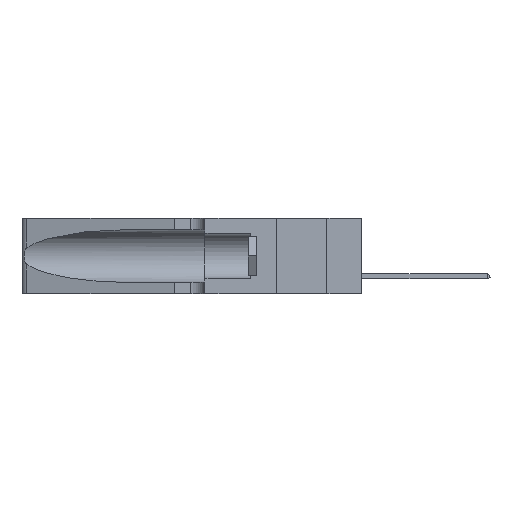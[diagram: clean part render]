
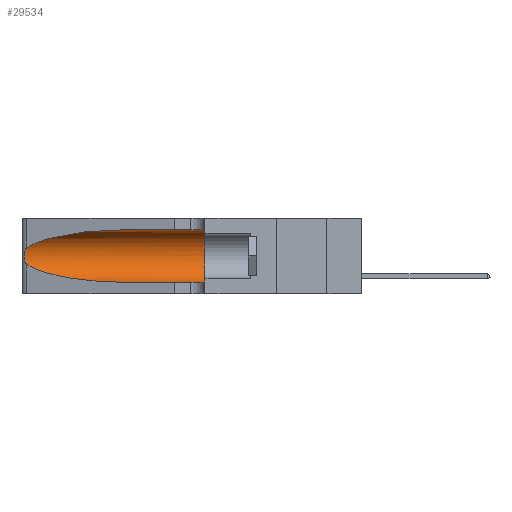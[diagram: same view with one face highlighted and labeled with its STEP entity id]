
A CAD part, left-side view. The second image highlights one B-rep face of the part: STEP entity #29534.
In plain terms, the highlighted cylindrical face has radius 3.308 mm (diameter 6.617 mm), a partial arc.
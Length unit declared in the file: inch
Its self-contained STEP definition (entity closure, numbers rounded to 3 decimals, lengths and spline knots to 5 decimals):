
#779 = EDGE_LOOP ( 'NONE', ( #20806, #25871, #9579, #47279, #19817, #12776 ) ) ;
#1622 = DIRECTION ( 'NONE',  ( 0., -1., 0. ) ) ;
#2119 = CARTESIAN_POINT ( 'NONE',  ( 0.1305, 1.61858, 0.05475 ) ) ;
#2508 =( BOUNDED_CURVE ( )  B_SPLINE_CURVE ( 3, ( #24202, #8757, #34738, #9250 ),
 .UNSPECIFIED., .F., .F. ) 
 B_SPLINE_CURVE_WITH_KNOTS ( ( 4, 4 ),
 ( 1.5708, 2.84003 ),
 .UNSPECIFIED. ) 
 CURVE ( )  GEOMETRIC_REPRESENTATION_ITEM ( )  RATIONAL_B_SPLINE_CURVE ( ( 1., 0.87, 0.87, 1. ) ) 
 REPRESENTATION_ITEM ( '' )  );
#2525 = CARTESIAN_POINT ( 'NONE',  ( 0.26075, 1.23896, 0.19203 ) ) ;
#3114 = CARTESIAN_POINT ( 'NONE',  ( 0.25487, 1.22718, 0.14631 ) ) ;
#3677 = CARTESIAN_POINT ( 'NONE',  ( 0.1305, 0.35, 0.31525 ) ) ;
#4742 = CARTESIAN_POINT ( 'NONE',  ( 0.1305, 0.72297, 0.05475 ) ) ;
#4957 = LINE ( 'NONE', #36400, #30620 ) ;
#6187 = AXIS2_PLACEMENT_3D ( 'NONE', #39649, #39001, #13636 ) ;
#6222 = CARTESIAN_POINT ( 'NONE',  ( 0.25856, 1.23593, 0.16098 ) ) ;
#8757 = CARTESIAN_POINT ( 'NONE',  ( 0.18966, 0.96281, 0.31525 ) ) ;
#9161 = EDGE_CURVE ( 'NONE', #24756, #40914, #35566, .T. ) ;
#9250 = CARTESIAN_POINT ( 'NONE',  ( 0.25487, 1.22718, 0.22369 ) ) ;
#9579 = ORIENTED_EDGE ( 'NONE', *, *, #41600, .T. ) ;
#10111 = VECTOR ( 'NONE', #1622, 39.37008 ) ;
#10436 = CARTESIAN_POINT ( 'NONE',  ( 0.25555, 1.22993, 0.14849 ) ) ;
#11319 = EDGE_CURVE ( 'NONE', #23641, #26205, #39185, .T. ) ;
#11950 = CIRCLE ( 'NONE', #30558, 0.13025 ) ;
#12776 = ORIENTED_EDGE ( 'NONE', *, *, #42038, .F. ) ;
#13636 = DIRECTION ( 'NONE',  ( 0., 0., -1. ) ) ;
#13825 = CARTESIAN_POINT ( 'NONE',  ( 0.25789, 1.23486, 0.15765 ) ) ;
#16120 =( BOUNDED_CURVE ( )  B_SPLINE_CURVE ( 3, ( #3114, #36759, #21975, #47924 ),
 .UNSPECIFIED., .F., .T. ) 
 B_SPLINE_CURVE_WITH_KNOTS ( ( 4, 4 ),
 ( 3.44316, 4.71239 ),
 .UNSPECIFIED. ) 
 CURVE ( )  GEOMETRIC_REPRESENTATION_ITEM ( )  RATIONAL_B_SPLINE_CURVE ( ( 1., 0.87, 0.87, 1. ) ) 
 REPRESENTATION_ITEM ( '' )  );
#17600 = CARTESIAN_POINT ( 'NONE',  ( 0.26017, 1.23833, 0.17102 ) ) ;
#18816 = VERTEX_POINT ( 'NONE', #31425 ) ;
#19817 = ORIENTED_EDGE ( 'NONE', *, *, #41970, .F. ) ;
#20806 = ORIENTED_EDGE ( 'NONE', *, *, #33502, .T. ) ;
#21626 = CYLINDRICAL_SURFACE ( 'NONE', #6187, 0.13025 ) ;
#21975 = CARTESIAN_POINT ( 'NONE',  ( 0.18966, 0.96281, 0.05475 ) ) ;
#22194 = CARTESIAN_POINT ( 'NONE',  ( 0.25487, 1.22718, 0.22369 ) ) ;
#23641 = VERTEX_POINT ( 'NONE', #4742 ) ;
#24202 = CARTESIAN_POINT ( 'NONE',  ( 0.1305, 0.72297, 0.31525 ) ) ;
#24743 = CARTESIAN_POINT ( 'NONE',  ( 0.25787, 1.23484, 0.2124 ) ) ;
#24756 = VERTEX_POINT ( 'NONE', #37142 ) ;
#25225 = CARTESIAN_POINT ( 'NONE',  ( 0.25487, 1.22718, 0.14631 ) ) ;
#25772 = CARTESIAN_POINT ( 'NONE',  ( 0.25555, 1.22994, 0.2215 ) ) ;
#25871 = ORIENTED_EDGE ( 'NONE', *, *, #9161, .T. ) ;
#26199 = VERTEX_POINT ( 'NONE', #3677 ) ;
#26205 = VERTEX_POINT ( 'NONE', #45407 ) ;
#28542 = CARTESIAN_POINT ( 'NONE',  ( 0.26075, 1.23896, 0.178 ) ) ;
#29534 = ADVANCED_FACE ( 'NONE', ( #36775 ), #21626, .F. ) ;
#30558 = AXIS2_PLACEMENT_3D ( 'NONE', #31722, #46252, #45922 ) ;
#30620 = VECTOR ( 'NONE', #40089, 39.37008 ) ;
#31425 = CARTESIAN_POINT ( 'NONE',  ( 0.1305, 0.72297, 0.31525 ) ) ;
#31464 = CARTESIAN_POINT ( 'NONE',  ( 0.25639, 1.23184, 0.21858 ) ) ;
#31722 = CARTESIAN_POINT ( 'NONE',  ( 0.1305, 0.35, 0.185 ) ) ;
#32266 = CARTESIAN_POINT ( 'NONE',  ( 0.25639, 1.23186, 0.15144 ) ) ;
#33502 = EDGE_CURVE ( 'NONE', #18816, #24756, #2508, .T. ) ;
#34738 = CARTESIAN_POINT ( 'NONE',  ( 0.2373, 1.15595, 0.28018 ) ) ;
#35566 = B_SPLINE_CURVE_WITH_KNOTS ( 'NONE', 3,
 ( #22194, #25772, #31464, #24743, #39995, #39854, #2525, #28542, #17600, #6222, #13825, #32266, #10436, #25225 ),
 .UNSPECIFIED., .F., .F.,
 ( 4, 2, 2, 2, 2, 2, 4 ),
 ( 0., 0.00027, 0.00053, 0.00107, 0.0016, 0.00187, 0.00214 ),
 .UNSPECIFIED. ) ;
#36400 = CARTESIAN_POINT ( 'NONE',  ( 0.1305, 1.61858, 0.31525 ) ) ;
#36759 = CARTESIAN_POINT ( 'NONE',  ( 0.2373, 1.15595, 0.08982 ) ) ;
#36775 = FACE_OUTER_BOUND ( 'NONE', #779, .T. ) ;
#37142 = CARTESIAN_POINT ( 'NONE',  ( 0.25487, 1.22718, 0.22369 ) ) ;
#39001 = DIRECTION ( 'NONE',  ( 0., -1., 0. ) ) ;
#39185 = LINE ( 'NONE', #2119, #10111 ) ;
#39649 = CARTESIAN_POINT ( 'NONE',  ( 0.1305, 1.61858, 0.185 ) ) ;
#39854 = CARTESIAN_POINT ( 'NONE',  ( 0.26018, 1.23835, 0.19895 ) ) ;
#39995 = CARTESIAN_POINT ( 'NONE',  ( 0.25854, 1.2359, 0.20912 ) ) ;
#40089 = DIRECTION ( 'NONE',  ( 0., -1., 0. ) ) ;
#40243 = CARTESIAN_POINT ( 'NONE',  ( 0.25487, 1.22718, 0.14631 ) ) ;
#40914 = VERTEX_POINT ( 'NONE', #40243 ) ;
#41600 = EDGE_CURVE ( 'NONE', #40914, #23641, #16120, .T. ) ;
#41970 = EDGE_CURVE ( 'NONE', #26199, #26205, #11950, .T. ) ;
#42038 = EDGE_CURVE ( 'NONE', #18816, #26199, #4957, .T. ) ;
#45407 = CARTESIAN_POINT ( 'NONE',  ( 0.1305, 0.35, 0.05475 ) ) ;
#45922 = DIRECTION ( 'NONE',  ( 0., 0., 1. ) ) ;
#46252 = DIRECTION ( 'NONE',  ( 0., 1., 0. ) ) ;
#47279 = ORIENTED_EDGE ( 'NONE', *, *, #11319, .T. ) ;
#47924 = CARTESIAN_POINT ( 'NONE',  ( 0.1305, 0.72297, 0.05475 ) ) ;
